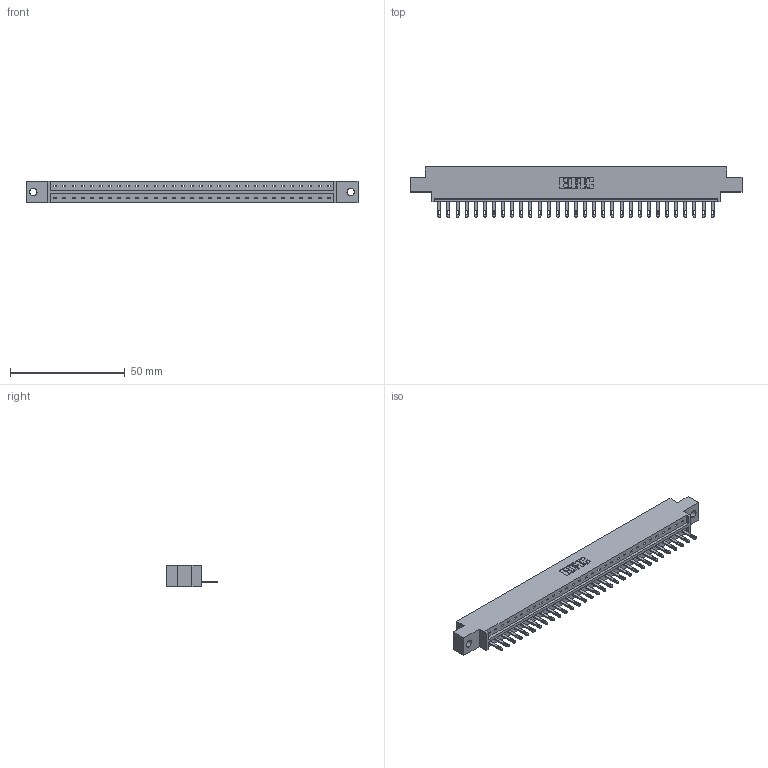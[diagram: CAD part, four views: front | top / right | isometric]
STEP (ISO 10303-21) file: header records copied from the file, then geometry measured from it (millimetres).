
FILE_DESCRIPTION (( 'STEP AP203' ), '1' );
FILE_NAME ('833-031-500-602.STEP', '2020-06-02T14:51:46', ( '' ), ( '' ), 'SwSTEP 2.0', 'SolidWorks 2020', '' );
FILE_SCHEMA (( 'CONFIG_CONTROL_DESIGN' ));
Length unit declared in the file: inch
Products named in the file (3): 833 Part_Offset - .128 Dia; 345-292-001_345-293-100; 833-031-500-602
Assembly tree (32 placements, depth 2):
  833-031-500-602
    833 Part_Offset - .128 Dia
    345-292-001_345-293-100  x31
Bounding box: 144.37 x 21.85 x 9.4 mm (x, y, z)
Volume: 14188.2 mm3; surface area: 15280.4 mm2
Topology: 32 solids, 32 shells, 1792 faces, 5531 edges, 3686 vertices
Faces by surface type: plane 1190, cylinder 602
Entity records: 20439 total; most frequent: CARTESIAN_POINT 3535, ORIENTED_EDGE 3502, DIRECTION 3005, EDGE_CURVE 1751, LINE 1619, VECTOR 1619, VERTEX_POINT 1166, AXIS2_PLACEMENT_3D 693
